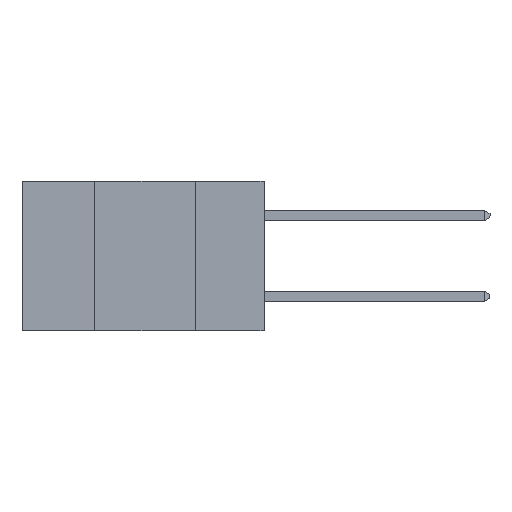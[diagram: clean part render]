
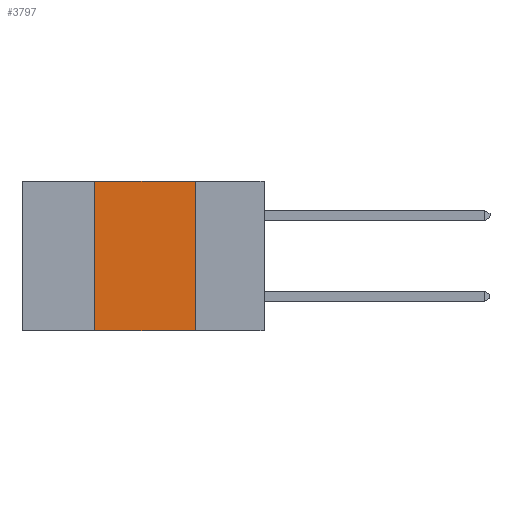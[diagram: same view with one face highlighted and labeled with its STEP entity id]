
A CAD part, left-side view. The second image highlights one B-rep face of the part: STEP entity #3797.
In plain terms, the highlighted planar face has unit normal (-1, 0, 0).
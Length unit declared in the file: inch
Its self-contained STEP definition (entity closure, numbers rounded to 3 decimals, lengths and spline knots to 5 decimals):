
#316 = VERTEX_POINT ( 'NONE', #10816 ) ;
#1110 = DIRECTION ( 'NONE',  ( 0., -1., 0. ) ) ;
#1475 = ORIENTED_EDGE ( 'NONE', *, *, #4316, .F. ) ;
#1564 = VERTEX_POINT ( 'NONE', #1831 ) ;
#1817 = DIRECTION ( 'NONE',  ( 0., -1., 0. ) ) ;
#1831 = CARTESIAN_POINT ( 'NONE',  ( 0., 0.17, -0.37 ) ) ;
#1898 = VECTOR ( 'NONE', #10291, 39.37008 ) ;
#1916 = ORIENTED_EDGE ( 'NONE', *, *, #4159, .F. ) ;
#2034 = LINE ( 'NONE', #8968, #11301 ) ;
#2740 = LINE ( 'NONE', #11373, #6979 ) ;
#3797 = ADVANCED_FACE ( 'NONE', ( #9011 ), #9172, .F. ) ;
#4114 = EDGE_CURVE ( 'NONE', #316, #7004, #10675, .T. ) ;
#4159 = EDGE_CURVE ( 'NONE', #9736, #1564, #7907, .T. ) ;
#4316 = EDGE_CURVE ( 'NONE', #7004, #9736, #2740, .T. ) ;
#4448 = EDGE_CURVE ( 'NONE', #316, #1564, #2034, .T. ) ;
#4828 = AXIS2_PLACEMENT_3D ( 'NONE', #9148, #6290, #6183 ) ;
#4834 = CARTESIAN_POINT ( 'NONE',  ( 0., 0.42, 0. ) ) ;
#5664 = VECTOR ( 'NONE', #7458, 39.37008 ) ;
#6183 = DIRECTION ( 'NONE',  ( 0., 0., -1. ) ) ;
#6290 = DIRECTION ( 'NONE',  ( 1., 0., 0. ) ) ;
#6979 = VECTOR ( 'NONE', #1110, 39.37008 ) ;
#7004 = VERTEX_POINT ( 'NONE', #8452 ) ;
#7425 = CARTESIAN_POINT ( 'NONE',  ( 0., 0.17, 0. ) ) ;
#7458 = DIRECTION ( 'NONE',  ( 0., 0., -1. ) ) ;
#7907 = LINE ( 'NONE', #7425, #5664 ) ;
#8452 = CARTESIAN_POINT ( 'NONE',  ( 0., 0.42, 0. ) ) ;
#8968 = CARTESIAN_POINT ( 'NONE',  ( 0., 0.6, -0.37 ) ) ;
#9011 = FACE_OUTER_BOUND ( 'NONE', #11162, .T. ) ;
#9148 = CARTESIAN_POINT ( 'NONE',  ( 0., 0.6, 0. ) ) ;
#9172 = PLANE ( 'NONE',  #4828 ) ;
#9736 = VERTEX_POINT ( 'NONE', #11215 ) ;
#10291 = DIRECTION ( 'NONE',  ( 0., 0., 1. ) ) ;
#10303 = ORIENTED_EDGE ( 'NONE', *, *, #4448, .T. ) ;
#10560 = ORIENTED_EDGE ( 'NONE', *, *, #4114, .F. ) ;
#10675 = LINE ( 'NONE', #4834, #1898 ) ;
#10816 = CARTESIAN_POINT ( 'NONE',  ( 0., 0.42, -0.37 ) ) ;
#11162 = EDGE_LOOP ( 'NONE', ( #1916, #1475, #10560, #10303 ) ) ;
#11215 = CARTESIAN_POINT ( 'NONE',  ( 0., 0.17, 0. ) ) ;
#11301 = VECTOR ( 'NONE', #1817, 39.37008 ) ;
#11373 = CARTESIAN_POINT ( 'NONE',  ( 0., 0.6, 0. ) ) ;
